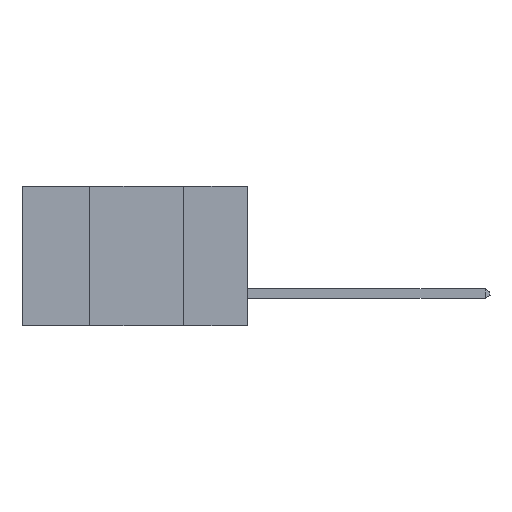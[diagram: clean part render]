
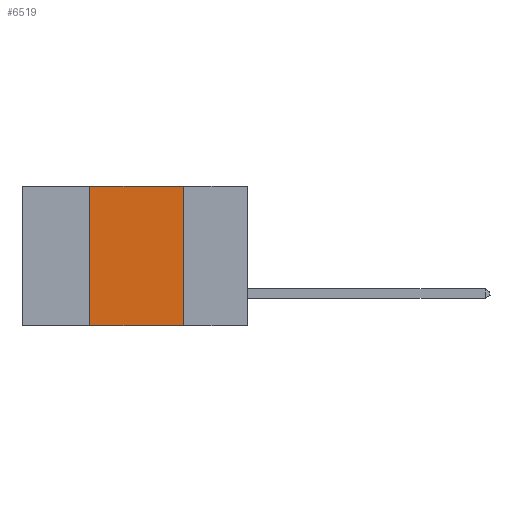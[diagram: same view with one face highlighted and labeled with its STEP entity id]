
A CAD part, left-side view. The second image highlights one B-rep face of the part: STEP entity #6519.
In plain terms, the highlighted planar face has unit normal (-1, 0, 0).
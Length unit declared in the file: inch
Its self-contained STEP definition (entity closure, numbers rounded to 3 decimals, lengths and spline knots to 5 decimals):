
#345 = VERTEX_POINT ( 'NONE', #2489 ) ;
#603 = VECTOR ( 'NONE', #8765, 39.37008 ) ;
#832 = AXIS2_PLACEMENT_3D ( 'NONE', #965, #9796, #9869 ) ;
#965 = CARTESIAN_POINT ( 'NONE',  ( 0., 0.6, 0. ) ) ;
#1063 = LINE ( 'NONE', #7907, #9405 ) ;
#1486 = LINE ( 'NONE', #6186, #603 ) ;
#1554 = CARTESIAN_POINT ( 'NONE',  ( 0., 0.17, -0.37 ) ) ;
#1875 = EDGE_LOOP ( 'NONE', ( #6911, #7317, #7781, #8998 ) ) ;
#2097 = EDGE_CURVE ( 'NONE', #6252, #8537, #1486, .T. ) ;
#2359 = VECTOR ( 'NONE', #10257, 39.37008 ) ;
#2489 = CARTESIAN_POINT ( 'NONE',  ( 0., 0.42, 0. ) ) ;
#2679 = CARTESIAN_POINT ( 'NONE',  ( 0., 0.6, -0.37 ) ) ;
#3498 = CARTESIAN_POINT ( 'NONE',  ( 0., 0.42, -0.37 ) ) ;
#3708 = EDGE_CURVE ( 'NONE', #6813, #345, #1063, .T. ) ;
#3773 = EDGE_CURVE ( 'NONE', #345, #6252, #4010, .T. ) ;
#3954 = LINE ( 'NONE', #2679, #9594 ) ;
#4010 = LINE ( 'NONE', #8602, #2359 ) ;
#4600 = DIRECTION ( 'NONE',  ( 0., 0., 1. ) ) ;
#5111 = PLANE ( 'NONE',  #832 ) ;
#5382 = EDGE_CURVE ( 'NONE', #6813, #8537, #3954, .T. ) ;
#6186 = CARTESIAN_POINT ( 'NONE',  ( 0., 0.17, 0. ) ) ;
#6252 = VERTEX_POINT ( 'NONE', #9326 ) ;
#6519 = ADVANCED_FACE ( 'NONE', ( #7325 ), #5111, .F. ) ;
#6813 = VERTEX_POINT ( 'NONE', #3498 ) ;
#6911 = ORIENTED_EDGE ( 'NONE', *, *, #2097, .F. ) ;
#7317 = ORIENTED_EDGE ( 'NONE', *, *, #3773, .F. ) ;
#7325 = FACE_OUTER_BOUND ( 'NONE', #1875, .T. ) ;
#7781 = ORIENTED_EDGE ( 'NONE', *, *, #3708, .F. ) ;
#7907 = CARTESIAN_POINT ( 'NONE',  ( 0., 0.42, 0. ) ) ;
#8276 = DIRECTION ( 'NONE',  ( 0., -1., 0. ) ) ;
#8537 = VERTEX_POINT ( 'NONE', #1554 ) ;
#8602 = CARTESIAN_POINT ( 'NONE',  ( 0., 0.6, 0. ) ) ;
#8765 = DIRECTION ( 'NONE',  ( 0., 0., -1. ) ) ;
#8998 = ORIENTED_EDGE ( 'NONE', *, *, #5382, .T. ) ;
#9326 = CARTESIAN_POINT ( 'NONE',  ( 0., 0.17, 0. ) ) ;
#9405 = VECTOR ( 'NONE', #4600, 39.37008 ) ;
#9594 = VECTOR ( 'NONE', #8276, 39.37008 ) ;
#9796 = DIRECTION ( 'NONE',  ( 1., 0., 0. ) ) ;
#9869 = DIRECTION ( 'NONE',  ( 0., 0., -1. ) ) ;
#10257 = DIRECTION ( 'NONE',  ( 0., -1., 0. ) ) ;
